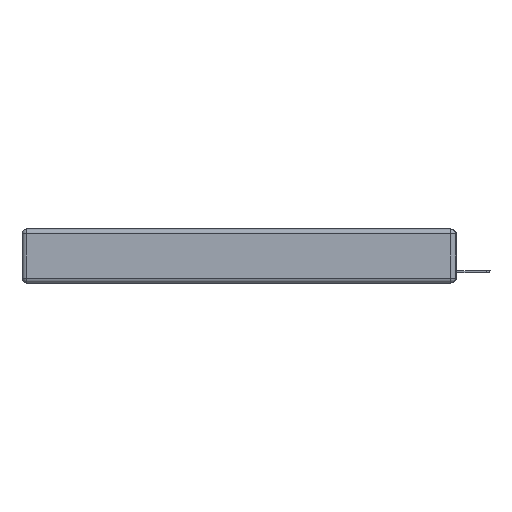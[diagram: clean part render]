
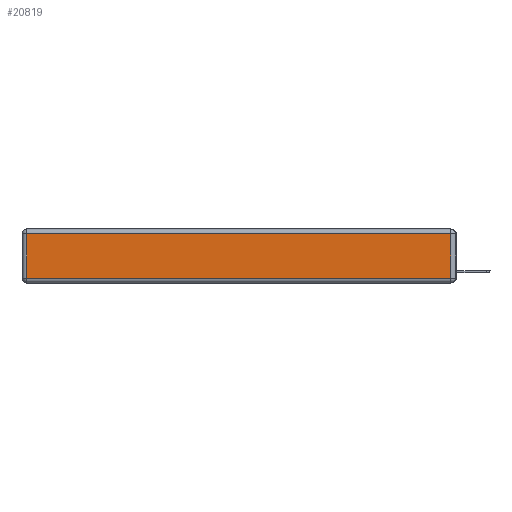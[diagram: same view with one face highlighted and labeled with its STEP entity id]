
A CAD part, left-side view. The second image highlights one B-rep face of the part: STEP entity #20819.
In plain terms, the highlighted planar face has unit normal (-1, 0, 0).
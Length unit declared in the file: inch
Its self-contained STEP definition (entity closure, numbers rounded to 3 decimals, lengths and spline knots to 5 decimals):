
#2144 = CARTESIAN_POINT ( 'NONE',  ( 0., 0.03, -0.313 ) ) ;
#2167 = VERTEX_POINT ( 'NONE', #3907 ) ;
#2726 = EDGE_CURVE ( 'NONE', #2167, #22143, #4840, .T. ) ;
#2982 = CARTESIAN_POINT ( 'NONE',  ( 0., 0., -0.343 ) ) ;
#3907 = CARTESIAN_POINT ( 'NONE',  ( 0., 0.03, -0.03 ) ) ;
#4840 = LINE ( 'NONE', #17595, #16731 ) ;
#4964 = DIRECTION ( 'NONE',  ( 0., 1., 0. ) ) ;
#6755 = ORIENTED_EDGE ( 'NONE', *, *, #2726, .T. ) ;
#6981 = AXIS2_PLACEMENT_3D ( 'NONE', #2982, #11531, #20097 ) ;
#7220 = CARTESIAN_POINT ( 'NONE',  ( 0., 2.72, -0.313 ) ) ;
#7602 = ORIENTED_EDGE ( 'NONE', *, *, #25414, .T. ) ;
#7803 = DIRECTION ( 'NONE',  ( 0., -1., 0. ) ) ;
#8872 = EDGE_LOOP ( 'NONE', ( #12568, #7602, #6755, #13373 ) ) ;
#9490 = CARTESIAN_POINT ( 'NONE',  ( 0., 0.03, -0.343 ) ) ;
#10069 = DIRECTION ( 'NONE',  ( 0., 0., -1. ) ) ;
#11531 = DIRECTION ( 'NONE',  ( -1., 0., 0. ) ) ;
#12042 = CARTESIAN_POINT ( 'NONE',  ( 0., 2.72, -0.343 ) ) ;
#12568 = ORIENTED_EDGE ( 'NONE', *, *, #12747, .T. ) ;
#12747 = EDGE_CURVE ( 'NONE', #27559, #24681, #20878, .T. ) ;
#13373 = ORIENTED_EDGE ( 'NONE', *, *, #26643, .T. ) ;
#13485 = VECTOR ( 'NONE', #26908, 39.37008 ) ;
#14606 = CARTESIAN_POINT ( 'NONE',  ( 0., 2.72, -0.03 ) ) ;
#16731 = VECTOR ( 'NONE', #4964, 39.37008 ) ;
#17595 = CARTESIAN_POINT ( 'NONE',  ( 0., 2.75, -0.03 ) ) ;
#18403 = FACE_OUTER_BOUND ( 'NONE', #8872, .T. ) ;
#20097 = DIRECTION ( 'NONE',  ( 0., 0., 1. ) ) ;
#20819 = ADVANCED_FACE ( 'NONE', ( #18403 ), #22208, .T. ) ;
#20878 = LINE ( 'NONE', #27032, #26980 ) ;
#22143 = VERTEX_POINT ( 'NONE', #14606 ) ;
#22208 = PLANE ( 'NONE',  #6981 ) ;
#22472 = VECTOR ( 'NONE', #10069, 39.37008 ) ;
#24548 = LINE ( 'NONE', #12042, #22472 ) ;
#24681 = VERTEX_POINT ( 'NONE', #2144 ) ;
#25414 = EDGE_CURVE ( 'NONE', #24681, #2167, #27049, .T. ) ;
#26643 = EDGE_CURVE ( 'NONE', #22143, #27559, #24548, .T. ) ;
#26908 = DIRECTION ( 'NONE',  ( 0., 0., 1. ) ) ;
#26980 = VECTOR ( 'NONE', #7803, 39.37008 ) ;
#27032 = CARTESIAN_POINT ( 'NONE',  ( 0., 0., -0.313 ) ) ;
#27049 = LINE ( 'NONE', #9490, #13485 ) ;
#27559 = VERTEX_POINT ( 'NONE', #7220 ) ;
